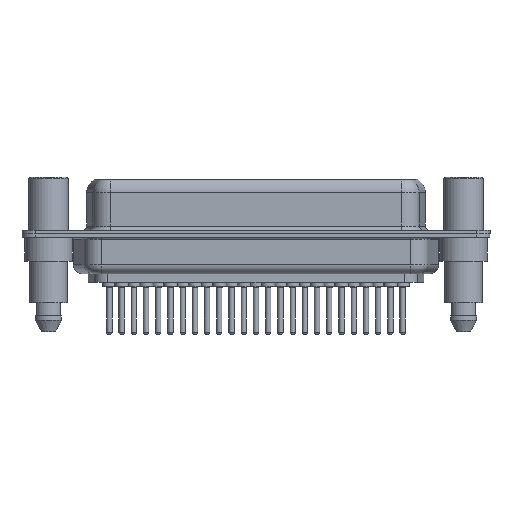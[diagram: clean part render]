
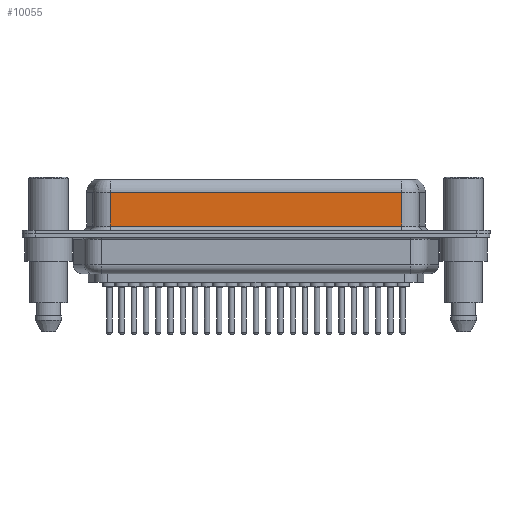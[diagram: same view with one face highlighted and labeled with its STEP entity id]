
A CAD part, front view. The second image highlights one B-rep face of the part: STEP entity #10055.
In plain terms, the highlighted planar face has unit normal (0, -1, 0).
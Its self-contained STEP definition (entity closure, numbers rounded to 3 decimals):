
#8 = ORIENTED_EDGE ( 'NONE', *, *, #13812, .T. ) ;
#139 = EDGE_LOOP ( 'NONE', ( #20192, #5450, #8, #12866 ) ) ;
#1659 = VECTOR ( 'NONE', #1667, 1000. ) ;
#1667 = DIRECTION ( 'NONE',  ( -1., 0., 0. ) ) ;
#2708 = EDGE_CURVE ( 'NONE', #8429, #15892, #10591, .T. ) ;
#2720 = VECTOR ( 'NONE', #5307, 1000. ) ;
#4643 = CARTESIAN_POINT ( 'NONE',  ( 7.013, -3.95, 6.4 ) ) ;
#5155 = CARTESIAN_POINT ( 'NONE',  ( 40.037, -3.95, 6.4 ) ) ;
#5307 = DIRECTION ( 'NONE',  ( 1., 0., 0. ) ) ;
#5450 = ORIENTED_EDGE ( 'NONE', *, *, #7721, .T. ) ;
#6949 = CARTESIAN_POINT ( 'NONE',  ( 40.037, -3.95, 0.9 ) ) ;
#7300 = DIRECTION ( 'NONE',  ( 0., 1., 0. ) ) ;
#7721 = EDGE_CURVE ( 'NONE', #17127, #22190, #22128, .T. ) ;
#8429 = VERTEX_POINT ( 'NONE', #20459 ) ;
#9198 = DIRECTION ( 'NONE',  ( 0., 0., -1. ) ) ;
#9375 = EDGE_CURVE ( 'NONE', #17127, #15892, #17589, .T. ) ;
#10055 = ADVANCED_FACE ( 'NONE', ( #14243 ), #15939, .F. ) ;
#10591 = LINE ( 'NONE', #15750, #2720 ) ;
#10789 = VECTOR ( 'NONE', #9198, 1000. ) ;
#12015 = DIRECTION ( 'NONE',  ( 0., 0., 1. ) ) ;
#12544 = DIRECTION ( 'NONE',  ( 0., 0., -1. ) ) ;
#12866 = ORIENTED_EDGE ( 'NONE', *, *, #2708, .T. ) ;
#13159 = VECTOR ( 'NONE', #12544, 1000. ) ;
#13812 = EDGE_CURVE ( 'NONE', #22190, #8429, #21203, .T. ) ;
#14243 = FACE_OUTER_BOUND ( 'NONE', #139, .T. ) ;
#14556 = CARTESIAN_POINT ( 'NONE',  ( 40.037, -3.95, 6.4 ) ) ;
#15750 = CARTESIAN_POINT ( 'NONE',  ( 40.037, -3.95, 0.9 ) ) ;
#15892 = VERTEX_POINT ( 'NONE', #6949 ) ;
#15939 = PLANE ( 'NONE',  #16403 ) ;
#16403 = AXIS2_PLACEMENT_3D ( 'NONE', #5155, #7300, #12015 ) ;
#17127 = VERTEX_POINT ( 'NONE', #19438 ) ;
#17281 = CARTESIAN_POINT ( 'NONE',  ( 40.037, -3.95, 4.65 ) ) ;
#17589 = LINE ( 'NONE', #14556, #13159 ) ;
#18641 = CARTESIAN_POINT ( 'NONE',  ( 7.013, -3.95, 4.65 ) ) ;
#19438 = CARTESIAN_POINT ( 'NONE',  ( 40.037, -3.95, 4.65 ) ) ;
#20192 = ORIENTED_EDGE ( 'NONE', *, *, #9375, .F. ) ;
#20459 = CARTESIAN_POINT ( 'NONE',  ( 7.013, -3.95, 0.9 ) ) ;
#21203 = LINE ( 'NONE', #4643, #10789 ) ;
#22128 = LINE ( 'NONE', #17281, #1659 ) ;
#22190 = VERTEX_POINT ( 'NONE', #18641 ) ;
